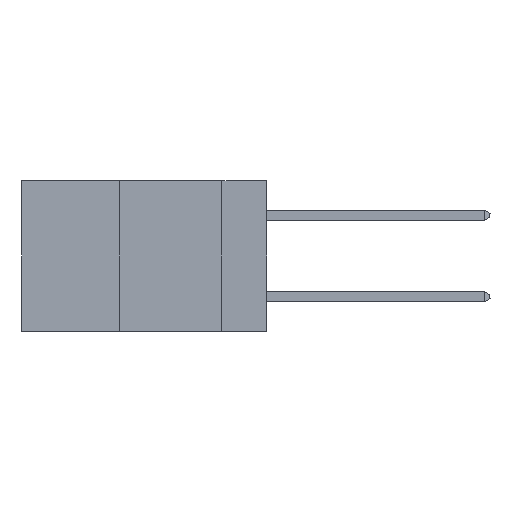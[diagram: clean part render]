
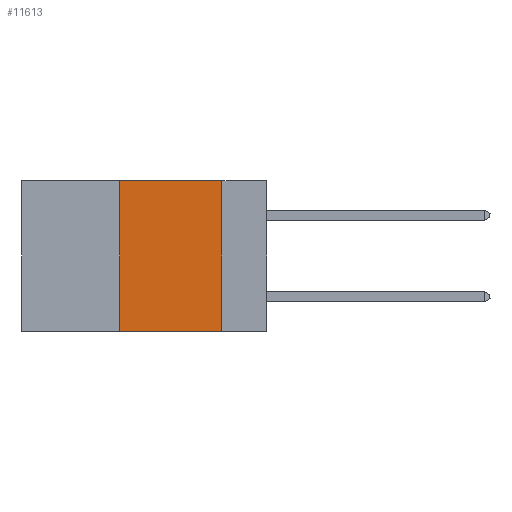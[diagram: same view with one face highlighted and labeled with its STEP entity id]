
A CAD part, left-side view. The second image highlights one B-rep face of the part: STEP entity #11613.
In plain terms, the highlighted planar face has unit normal (-1, 0, 0).
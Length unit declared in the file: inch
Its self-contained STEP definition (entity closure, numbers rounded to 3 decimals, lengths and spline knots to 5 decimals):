
#349 = CARTESIAN_POINT ( 'NONE',  ( 0., 0.6, 0. ) ) ;
#2602 = EDGE_CURVE ( 'NONE', #22086, #26060, #42359, .T. ) ;
#4605 = FACE_OUTER_BOUND ( 'NONE', #19470, .T. ) ;
#5424 = VECTOR ( 'NONE', #10693, 39.37008 ) ;
#5469 = CARTESIAN_POINT ( 'NONE',  ( 0., 0.36, 0. ) ) ;
#5783 = LINE ( 'NONE', #32998, #25545 ) ;
#6926 = CARTESIAN_POINT ( 'NONE',  ( 0., 0.6, -0.37 ) ) ;
#7277 = VECTOR ( 'NONE', #42004, 39.37008 ) ;
#10373 = AXIS2_PLACEMENT_3D ( 'NONE', #349, #22630, #45030 ) ;
#10693 = DIRECTION ( 'NONE',  ( 0., -1., 0. ) ) ;
#11613 = ADVANCED_FACE ( 'NONE', ( #4605 ), #33328, .F. ) ;
#14431 = EDGE_CURVE ( 'NONE', #30766, #22086, #5783, .T. ) ;
#14985 = CARTESIAN_POINT ( 'NONE',  ( 0., 0.11, 0. ) ) ;
#17699 = CARTESIAN_POINT ( 'NONE',  ( 0., 0.11, -0.37 ) ) ;
#18620 = EDGE_CURVE ( 'NONE', #27039, #26060, #32148, .T. ) ;
#19133 = VECTOR ( 'NONE', #19182, 39.37008 ) ;
#19182 = DIRECTION ( 'NONE',  ( 0., 0., -1. ) ) ;
#19355 = ORIENTED_EDGE ( 'NONE', *, *, #2602, .F. ) ;
#19470 = EDGE_LOOP ( 'NONE', ( #19355, #38201, #37732, #33111 ) ) ;
#22086 = VERTEX_POINT ( 'NONE', #37119 ) ;
#22630 = DIRECTION ( 'NONE',  ( 1., 0., 0. ) ) ;
#24147 = DIRECTION ( 'NONE',  ( 0., -1., 0. ) ) ;
#25196 = EDGE_CURVE ( 'NONE', #27039, #30766, #32850, .T. ) ;
#25545 = VECTOR ( 'NONE', #24147, 39.37008 ) ;
#26060 = VERTEX_POINT ( 'NONE', #17699 ) ;
#27039 = VERTEX_POINT ( 'NONE', #31553 ) ;
#30766 = VERTEX_POINT ( 'NONE', #45884 ) ;
#31553 = CARTESIAN_POINT ( 'NONE',  ( 0., 0.36, -0.37 ) ) ;
#32148 = LINE ( 'NONE', #6926, #5424 ) ;
#32850 = LINE ( 'NONE', #5469, #7277 ) ;
#32998 = CARTESIAN_POINT ( 'NONE',  ( 0., 0.6, 0. ) ) ;
#33111 = ORIENTED_EDGE ( 'NONE', *, *, #18620, .T. ) ;
#33328 = PLANE ( 'NONE',  #10373 ) ;
#37119 = CARTESIAN_POINT ( 'NONE',  ( 0., 0.11, 0. ) ) ;
#37732 = ORIENTED_EDGE ( 'NONE', *, *, #25196, .F. ) ;
#38201 = ORIENTED_EDGE ( 'NONE', *, *, #14431, .F. ) ;
#42004 = DIRECTION ( 'NONE',  ( 0., 0., 1. ) ) ;
#42359 = LINE ( 'NONE', #14985, #19133 ) ;
#45030 = DIRECTION ( 'NONE',  ( 0., 0., -1. ) ) ;
#45884 = CARTESIAN_POINT ( 'NONE',  ( 0., 0.36, 0. ) ) ;
